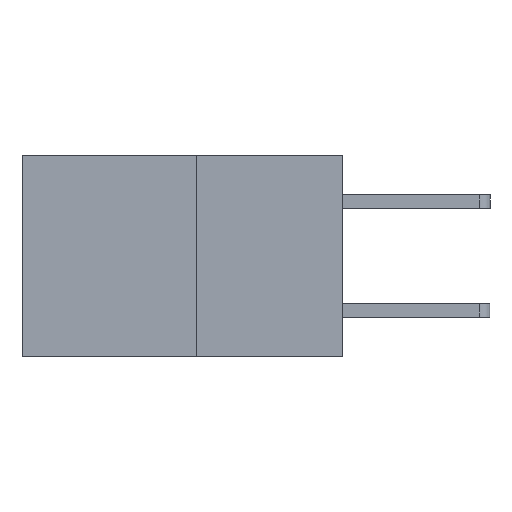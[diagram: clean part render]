
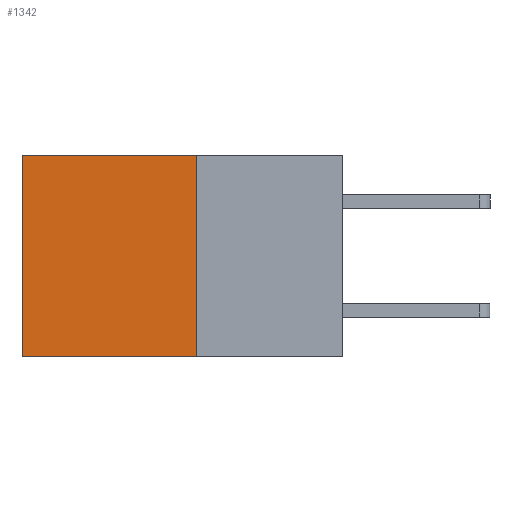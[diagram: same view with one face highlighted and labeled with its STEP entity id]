
A CAD part, left-side view. The second image highlights one B-rep face of the part: STEP entity #1342.
In plain terms, the highlighted planar face has unit normal (-1, 0, 0).
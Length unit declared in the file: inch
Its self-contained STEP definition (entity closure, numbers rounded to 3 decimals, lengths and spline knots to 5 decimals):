
#541 = VERTEX_POINT ( 'NONE', #749 ) ;
#736 = EDGE_CURVE ( 'NONE', #8732, #541, #4118, .T. ) ;
#749 = CARTESIAN_POINT ( 'NONE',  ( 0.277, 0.27, -0.37 ) ) ;
#881 = LINE ( 'NONE', #1659, #4433 ) ;
#1342 = ADVANCED_FACE ( 'NONE', ( #8266 ), #4481, .F. ) ;
#1659 = CARTESIAN_POINT ( 'NONE',  ( 0.277, 0.27, -0.37 ) ) ;
#2141 = CARTESIAN_POINT ( 'NONE',  ( 0.277, 0.59, -0.37 ) ) ;
#2505 = VECTOR ( 'NONE', #4217, 39.37008 ) ;
#2723 = VECTOR ( 'NONE', #3481, 39.37008 ) ;
#3179 = CARTESIAN_POINT ( 'NONE',  ( 0.277, 0.27, 0. ) ) ;
#3481 = DIRECTION ( 'NONE',  ( 0., 0., -1. ) ) ;
#3568 = CARTESIAN_POINT ( 'NONE',  ( 0.277, 0.27, 0. ) ) ;
#4041 = AXIS2_PLACEMENT_3D ( 'NONE', #7602, #7621, #7604 ) ;
#4118 = LINE ( 'NONE', #7608, #5702 ) ;
#4217 = DIRECTION ( 'NONE',  ( 0., 1., 0. ) ) ;
#4285 = LINE ( 'NONE', #3568, #2505 ) ;
#4433 = VECTOR ( 'NONE', #5699, 39.37008 ) ;
#4481 = PLANE ( 'NONE',  #4041 ) ;
#4613 = EDGE_CURVE ( 'NONE', #541, #8251, #881, .T. ) ;
#5428 = VERTEX_POINT ( 'NONE', #7724 ) ;
#5643 = ORIENTED_EDGE ( 'NONE', *, *, #4613, .F. ) ;
#5699 = DIRECTION ( 'NONE',  ( 0., 1., 0. ) ) ;
#5702 = VECTOR ( 'NONE', #8123, 39.37008 ) ;
#5845 = EDGE_CURVE ( 'NONE', #5428, #8251, #7792, .T. ) ;
#6056 = CARTESIAN_POINT ( 'NONE',  ( 0.277, 0.59, -0.37 ) ) ;
#6307 = EDGE_CURVE ( 'NONE', #8732, #5428, #4285, .T. ) ;
#7602 = CARTESIAN_POINT ( 'NONE',  ( 0.277, 0.27, -0.37 ) ) ;
#7604 = DIRECTION ( 'NONE',  ( 0., 0., -1. ) ) ;
#7608 = CARTESIAN_POINT ( 'NONE',  ( 0.277, 0.27, -0.37 ) ) ;
#7621 = DIRECTION ( 'NONE',  ( 1., 0., 0. ) ) ;
#7724 = CARTESIAN_POINT ( 'NONE',  ( 0.277, 0.59, 0. ) ) ;
#7792 = LINE ( 'NONE', #2141, #2723 ) ;
#7876 = ORIENTED_EDGE ( 'NONE', *, *, #736, .F. ) ;
#7966 = EDGE_LOOP ( 'NONE', ( #8063, #5643, #7876, #7973 ) ) ;
#7973 = ORIENTED_EDGE ( 'NONE', *, *, #6307, .T. ) ;
#8063 = ORIENTED_EDGE ( 'NONE', *, *, #5845, .T. ) ;
#8123 = DIRECTION ( 'NONE',  ( 0., 0., -1. ) ) ;
#8251 = VERTEX_POINT ( 'NONE', #6056 ) ;
#8266 = FACE_OUTER_BOUND ( 'NONE', #7966, .T. ) ;
#8732 = VERTEX_POINT ( 'NONE', #3179 ) ;
